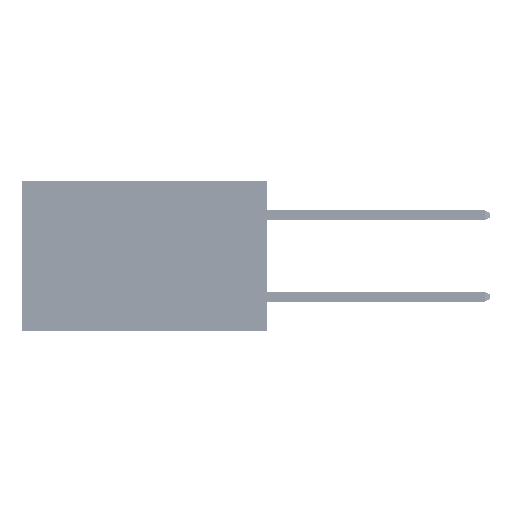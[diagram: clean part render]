
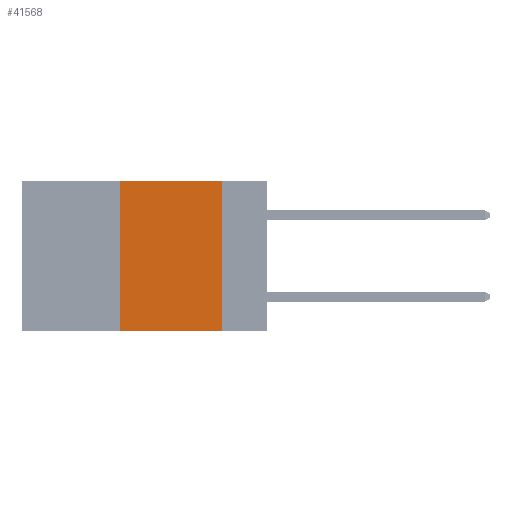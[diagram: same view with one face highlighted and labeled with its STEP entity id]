
A CAD part, left-side view. The second image highlights one B-rep face of the part: STEP entity #41568.
In plain terms, the highlighted planar face has unit normal (-1, 0, 0).
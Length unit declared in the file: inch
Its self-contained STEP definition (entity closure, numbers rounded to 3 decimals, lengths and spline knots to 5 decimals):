
#4716 = CARTESIAN_POINT ( 'NONE',  ( 0., 0.6, -0.37 ) ) ;
#4880 = EDGE_CURVE ( 'NONE', #18071, #17572, #29047, .T. ) ;
#6664 = VECTOR ( 'NONE', #40655, 39.37008 ) ;
#8386 = DIRECTION ( 'NONE',  ( 0., 0., -1. ) ) ;
#9116 = DIRECTION ( 'NONE',  ( 1., 0., 0. ) ) ;
#9897 = CARTESIAN_POINT ( 'NONE',  ( 0., 0.36, 0. ) ) ;
#9931 = EDGE_CURVE ( 'NONE', #18071, #47566, #42306, .T. ) ;
#12637 = CARTESIAN_POINT ( 'NONE',  ( 0., 0.6, 0. ) ) ;
#12760 = VECTOR ( 'NONE', #27539, 39.37008 ) ;
#16148 = CARTESIAN_POINT ( 'NONE',  ( 0., 0.11, 0. ) ) ;
#17572 = VERTEX_POINT ( 'NONE', #33332 ) ;
#18071 = VERTEX_POINT ( 'NONE', #19819 ) ;
#19819 = CARTESIAN_POINT ( 'NONE',  ( 0., 0.36, -0.37 ) ) ;
#22257 = ORIENTED_EDGE ( 'NONE', *, *, #9931, .T. ) ;
#24834 = EDGE_LOOP ( 'NONE', ( #29988, #29847, #39530, #22257 ) ) ;
#27539 = DIRECTION ( 'NONE',  ( 0., 0., -1. ) ) ;
#27929 = EDGE_CURVE ( 'NONE', #32108, #47566, #30584, .T. ) ;
#29047 = LINE ( 'NONE', #9897, #6664 ) ;
#29847 = ORIENTED_EDGE ( 'NONE', *, *, #47094, .F. ) ;
#29988 = ORIENTED_EDGE ( 'NONE', *, *, #27929, .F. ) ;
#30584 = LINE ( 'NONE', #16148, #12760 ) ;
#31516 = DIRECTION ( 'NONE',  ( 0., -1., 0. ) ) ;
#32108 = VERTEX_POINT ( 'NONE', #37856 ) ;
#33332 = CARTESIAN_POINT ( 'NONE',  ( 0., 0.36, 0. ) ) ;
#34720 = DIRECTION ( 'NONE',  ( 0., -1., 0. ) ) ;
#34801 = CARTESIAN_POINT ( 'NONE',  ( 0., 0.6, 0. ) ) ;
#36390 = CARTESIAN_POINT ( 'NONE',  ( 0., 0.11, -0.37 ) ) ;
#37856 = CARTESIAN_POINT ( 'NONE',  ( 0., 0.11, 0. ) ) ;
#38591 = LINE ( 'NONE', #34801, #47044 ) ;
#39530 = ORIENTED_EDGE ( 'NONE', *, *, #4880, .F. ) ;
#40655 = DIRECTION ( 'NONE',  ( 0., 0., 1. ) ) ;
#41568 = ADVANCED_FACE ( 'NONE', ( #47219 ), #43176, .F. ) ;
#42306 = LINE ( 'NONE', #4716, #48198 ) ;
#43176 = PLANE ( 'NONE',  #46018 ) ;
#46018 = AXIS2_PLACEMENT_3D ( 'NONE', #12637, #9116, #8386 ) ;
#47044 = VECTOR ( 'NONE', #31516, 39.37008 ) ;
#47094 = EDGE_CURVE ( 'NONE', #17572, #32108, #38591, .T. ) ;
#47219 = FACE_OUTER_BOUND ( 'NONE', #24834, .T. ) ;
#47566 = VERTEX_POINT ( 'NONE', #36390 ) ;
#48198 = VECTOR ( 'NONE', #34720, 39.37008 ) ;
